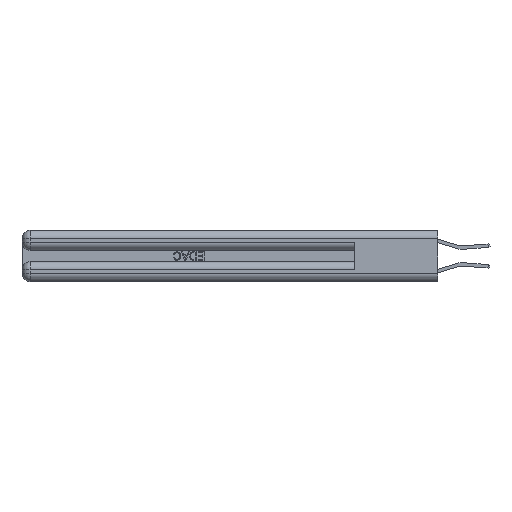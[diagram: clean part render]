
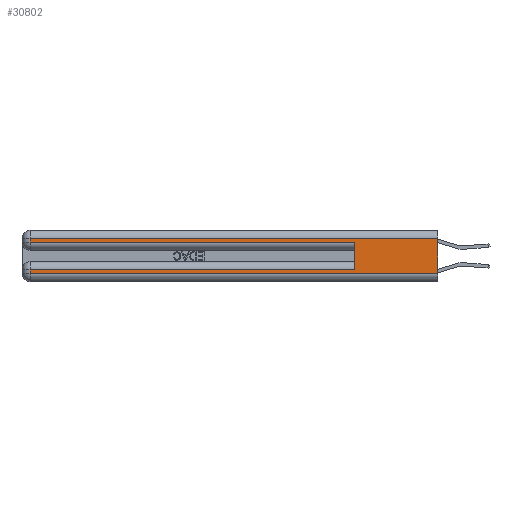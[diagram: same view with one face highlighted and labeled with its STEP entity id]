
A CAD part, left-side view. The second image highlights one B-rep face of the part: STEP entity #30802.
In plain terms, the highlighted planar face has unit normal (-1, 0, 0).
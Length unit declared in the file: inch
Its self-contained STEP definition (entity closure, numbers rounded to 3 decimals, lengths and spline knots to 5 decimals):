
#689 = DIRECTION ( 'NONE',  ( 1., 0., 0. ) ) ;
#1773 = EDGE_CURVE ( 'NONE', #2329, #6577, #28123, .T. ) ;
#2259 = EDGE_CURVE ( 'NONE', #31546, #8061, #23807, .T. ) ;
#2329 = VERTEX_POINT ( 'NONE', #16512 ) ;
#2634 = DIRECTION ( 'NONE',  ( 0., 0., -1. ) ) ;
#2844 = CARTESIAN_POINT ( 'NONE',  ( 0., 0., 0.37 ) ) ;
#3054 = ORIENTED_EDGE ( 'NONE', *, *, #11339, .F. ) ;
#4721 = ORIENTED_EDGE ( 'NONE', *, *, #1773, .T. ) ;
#5371 = LINE ( 'NONE', #9790, #31099 ) ;
#6143 = CARTESIAN_POINT ( 'NONE',  ( 0., 0.6, 0.085 ) ) ;
#6577 = VERTEX_POINT ( 'NONE', #23877 ) ;
#7215 = EDGE_CURVE ( 'NONE', #20768, #20096, #26923, .T. ) ;
#7434 = DIRECTION ( 'NONE',  ( 0., 0., -1. ) ) ;
#7805 = LINE ( 'NONE', #24965, #29595 ) ;
#7858 = VECTOR ( 'NONE', #31271, 39.37008 ) ;
#8061 = VERTEX_POINT ( 'NONE', #24558 ) ;
#8289 = DIRECTION ( 'NONE',  ( 0., -1., 0. ) ) ;
#9048 = VECTOR ( 'NONE', #7434, 39.37008 ) ;
#9790 = CARTESIAN_POINT ( 'NONE',  ( 0., 2.94, 0.37 ) ) ;
#10084 = EDGE_LOOP ( 'NONE', ( #3054, #4721, #12275, #31070, #15548, #28349, #17600, #26724 ) ) ;
#10912 = EDGE_CURVE ( 'NONE', #20768, #28520, #20058, .T. ) ;
#11339 = EDGE_CURVE ( 'NONE', #2329, #8061, #25102, .T. ) ;
#12275 = ORIENTED_EDGE ( 'NONE', *, *, #23261, .T. ) ;
#13029 = CARTESIAN_POINT ( 'NONE',  ( 0., 0.6, 0.285 ) ) ;
#13424 = CARTESIAN_POINT ( 'NONE',  ( 0., 0., 0.085 ) ) ;
#14588 = VECTOR ( 'NONE', #14970, 39.37008 ) ;
#14970 = DIRECTION ( 'NONE',  ( 0., 1., 0. ) ) ;
#15509 = PLANE ( 'NONE',  #26934 ) ;
#15548 = ORIENTED_EDGE ( 'NONE', *, *, #7215, .F. ) ;
#15568 = FACE_OUTER_BOUND ( 'NONE', #10084, .T. ) ;
#16512 = CARTESIAN_POINT ( 'NONE',  ( 0., 0., 0.31 ) ) ;
#17600 = ORIENTED_EDGE ( 'NONE', *, *, #27148, .T. ) ;
#17901 = CARTESIAN_POINT ( 'NONE',  ( 0., 2.94, 0.06 ) ) ;
#17919 = DIRECTION ( 'NONE',  ( 0., 1., 0. ) ) ;
#18024 = CARTESIAN_POINT ( 'NONE',  ( 0., 0., 0.37 ) ) ;
#18578 = CARTESIAN_POINT ( 'NONE',  ( 0., 0.6, 0.145 ) ) ;
#20058 = LINE ( 'NONE', #13424, #14588 ) ;
#20096 = VERTEX_POINT ( 'NONE', #13029 ) ;
#20240 = VERTEX_POINT ( 'NONE', #21079 ) ;
#20258 = DIRECTION ( 'NONE',  ( 0., -1., 0. ) ) ;
#20523 = DIRECTION ( 'NONE',  ( 0., 0., -1. ) ) ;
#20768 = VERTEX_POINT ( 'NONE', #6143 ) ;
#21079 = CARTESIAN_POINT ( 'NONE',  ( 0., 2.94, 0.285 ) ) ;
#22178 = CARTESIAN_POINT ( 'NONE',  ( 0., 2.94, 0.085 ) ) ;
#22396 = VECTOR ( 'NONE', #2634, 39.37008 ) ;
#23261 = EDGE_CURVE ( 'NONE', #6577, #20240, #5371, .T. ) ;
#23807 = LINE ( 'NONE', #25864, #24165 ) ;
#23877 = CARTESIAN_POINT ( 'NONE',  ( 0., 2.94, 0.31 ) ) ;
#24165 = VECTOR ( 'NONE', #8289, 39.37008 ) ;
#24558 = CARTESIAN_POINT ( 'NONE',  ( 0., 0., 0.06 ) ) ;
#24965 = CARTESIAN_POINT ( 'NONE',  ( 0., 0., 0.285 ) ) ;
#25102 = LINE ( 'NONE', #2844, #22396 ) ;
#25330 = DIRECTION ( 'NONE',  ( 0., 0., -1. ) ) ;
#25864 = CARTESIAN_POINT ( 'NONE',  ( 0., 0., 0.06 ) ) ;
#26165 = LINE ( 'NONE', #27417, #9048 ) ;
#26724 = ORIENTED_EDGE ( 'NONE', *, *, #2259, .T. ) ;
#26923 = LINE ( 'NONE', #18578, #7858 ) ;
#26934 = AXIS2_PLACEMENT_3D ( 'NONE', #18024, #689, #20523 ) ;
#27148 = EDGE_CURVE ( 'NONE', #28520, #31546, #26165, .T. ) ;
#27417 = CARTESIAN_POINT ( 'NONE',  ( 0., 2.94, 0.37 ) ) ;
#28063 = CARTESIAN_POINT ( 'NONE',  ( 0., 0., 0.31 ) ) ;
#28123 = LINE ( 'NONE', #28063, #29695 ) ;
#28349 = ORIENTED_EDGE ( 'NONE', *, *, #10912, .T. ) ;
#28520 = VERTEX_POINT ( 'NONE', #22178 ) ;
#29595 = VECTOR ( 'NONE', #20258, 39.37008 ) ;
#29695 = VECTOR ( 'NONE', #17919, 39.37008 ) ;
#30802 = ADVANCED_FACE ( 'NONE', ( #15568 ), #15509, .F. ) ;
#31070 = ORIENTED_EDGE ( 'NONE', *, *, #31212, .T. ) ;
#31099 = VECTOR ( 'NONE', #25330, 39.37008 ) ;
#31212 = EDGE_CURVE ( 'NONE', #20240, #20096, #7805, .T. ) ;
#31271 = DIRECTION ( 'NONE',  ( 0., 0., 1. ) ) ;
#31546 = VERTEX_POINT ( 'NONE', #17901 ) ;
